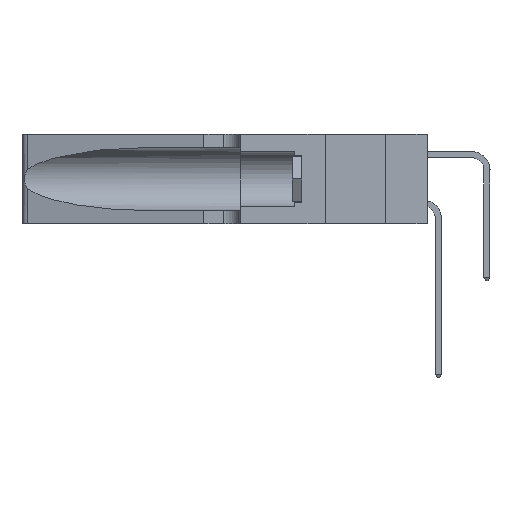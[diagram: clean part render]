
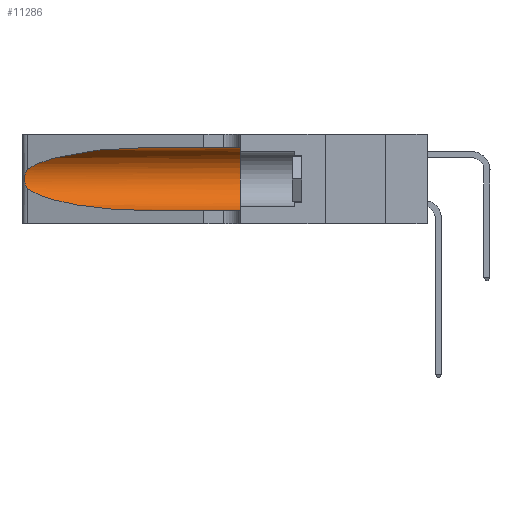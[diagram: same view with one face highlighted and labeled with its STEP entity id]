
A CAD part, left-side view. The second image highlights one B-rep face of the part: STEP entity #11286.
In plain terms, the highlighted cylindrical face has radius 3.308 mm (diameter 6.617 mm), a partial arc.
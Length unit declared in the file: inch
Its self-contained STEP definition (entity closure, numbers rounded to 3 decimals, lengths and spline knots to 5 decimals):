
#25 = ORIENTED_EDGE ( 'NONE', *, *, #1058, .F. ) ;
#624 = CARTESIAN_POINT ( 'NONE',  ( 0.18966, 0.96281, 0.31525 ) ) ;
#1058 = EDGE_CURVE ( 'NONE', #1945, #15296, #40654, .T. ) ;
#1204 = AXIS2_PLACEMENT_3D ( 'NONE', #14312, #21417, #45958 ) ;
#1569 = CARTESIAN_POINT ( 'NONE',  ( 0.25856, 1.23593, 0.16098 ) ) ;
#1945 = VERTEX_POINT ( 'NONE', #13621 ) ;
#3441 = LINE ( 'NONE', #28645, #9776 ) ;
#4288 = CARTESIAN_POINT ( 'NONE',  ( 0.1305, 0.72297, 0.31525 ) ) ;
#5263 = CARTESIAN_POINT ( 'NONE',  ( 0.25639, 1.23186, 0.15144 ) ) ;
#6060 = CARTESIAN_POINT ( 'NONE',  ( 0.1305, 0.72297, 0.05475 ) ) ;
#6554 =( BOUNDED_CURVE ( )  B_SPLINE_CURVE ( 3, ( #9323, #34014, #37522, #16544 ),
 .UNSPECIFIED., .F., .T. ) 
 B_SPLINE_CURVE_WITH_KNOTS ( ( 4, 4 ),
 ( 3.44316, 4.71239 ),
 .UNSPECIFIED. ) 
 CURVE ( )  GEOMETRIC_REPRESENTATION_ITEM ( )  RATIONAL_B_SPLINE_CURVE ( ( 1., 0.87, 0.87, 1. ) ) 
 REPRESENTATION_ITEM ( '' )  );
#7819 = EDGE_CURVE ( 'NONE', #11750, #35818, #38017, .T. ) ;
#8019 = CARTESIAN_POINT ( 'NONE',  ( 0.2373, 1.15595, 0.28018 ) ) ;
#8313 = ORIENTED_EDGE ( 'NONE', *, *, #36297, .T. ) ;
#8961 = CARTESIAN_POINT ( 'NONE',  ( 0.25487, 1.22718, 0.14631 ) ) ;
#9137 = DIRECTION ( 'NONE',  ( 0., 1., 0. ) ) ;
#9323 = CARTESIAN_POINT ( 'NONE',  ( 0.25487, 1.22718, 0.14631 ) ) ;
#9776 = VECTOR ( 'NONE', #11050, 39.37008 ) ;
#9978 = CYLINDRICAL_SURFACE ( 'NONE', #1204, 0.13025 ) ;
#10077 =( BOUNDED_CURVE ( )  B_SPLINE_CURVE ( 3, ( #4288, #624, #8019, #32741 ),
 .UNSPECIFIED., .F., .T. ) 
 B_SPLINE_CURVE_WITH_KNOTS ( ( 4, 4 ),
 ( 1.5708, 2.84003 ),
 .UNSPECIFIED. ) 
 CURVE ( )  GEOMETRIC_REPRESENTATION_ITEM ( )  RATIONAL_B_SPLINE_CURVE ( ( 1., 0.87, 0.87, 1. ) ) 
 REPRESENTATION_ITEM ( '' )  );
#10380 = CARTESIAN_POINT ( 'NONE',  ( 0.1305, 1.61858, 0.31525 ) ) ;
#11050 = DIRECTION ( 'NONE',  ( 0., -1., 0. ) ) ;
#11119 = FACE_OUTER_BOUND ( 'NONE', #19091, .T. ) ;
#11229 = EDGE_CURVE ( 'NONE', #44980, #1945, #32065, .T. ) ;
#11286 = ADVANCED_FACE ( 'NONE', ( #11119 ), #9978, .F. ) ;
#11750 = VERTEX_POINT ( 'NONE', #20463 ) ;
#12424 = CARTESIAN_POINT ( 'NONE',  ( 0.25487, 1.22718, 0.22369 ) ) ;
#13356 = VECTOR ( 'NONE', #28150, 39.37008 ) ;
#13621 = CARTESIAN_POINT ( 'NONE',  ( 0.1305, 0.35, 0.31525 ) ) ;
#14312 = CARTESIAN_POINT ( 'NONE',  ( 0.1305, 1.61858, 0.185 ) ) ;
#15296 = VERTEX_POINT ( 'NONE', #43865 ) ;
#15641 = AXIS2_PLACEMENT_3D ( 'NONE', #30321, #9137, #33827 ) ;
#16033 = CARTESIAN_POINT ( 'NONE',  ( 0.25854, 1.2359, 0.20912 ) ) ;
#16331 = CARTESIAN_POINT ( 'NONE',  ( 0.1305, 0.72297, 0.31525 ) ) ;
#16544 = CARTESIAN_POINT ( 'NONE',  ( 0.1305, 0.72297, 0.05475 ) ) ;
#17543 = CARTESIAN_POINT ( 'NONE',  ( 0.25487, 1.22718, 0.14631 ) ) ;
#19091 = EDGE_LOOP ( 'NONE', ( #41387, #35106, #8313, #22887, #25, #43897 ) ) ;
#19593 = CARTESIAN_POINT ( 'NONE',  ( 0.26075, 1.23896, 0.19203 ) ) ;
#20463 = CARTESIAN_POINT ( 'NONE',  ( 0.25487, 1.22718, 0.22369 ) ) ;
#21417 = DIRECTION ( 'NONE',  ( 0., -1., 0. ) ) ;
#22887 = ORIENTED_EDGE ( 'NONE', *, *, #39846, .T. ) ;
#23118 = CARTESIAN_POINT ( 'NONE',  ( 0.26017, 1.23833, 0.17102 ) ) ;
#26631 = CARTESIAN_POINT ( 'NONE',  ( 0.25789, 1.23486, 0.15765 ) ) ;
#28150 = DIRECTION ( 'NONE',  ( 0., -1., 0. ) ) ;
#28645 = CARTESIAN_POINT ( 'NONE',  ( 0.1305, 1.61858, 0.05475 ) ) ;
#30157 = CARTESIAN_POINT ( 'NONE',  ( 0.25555, 1.22993, 0.14849 ) ) ;
#30321 = CARTESIAN_POINT ( 'NONE',  ( 0.1305, 0.35, 0.185 ) ) ;
#31956 = EDGE_CURVE ( 'NONE', #44980, #11750, #10077, .T. ) ;
#32065 = LINE ( 'NONE', #10380, #13356 ) ;
#32253 = VERTEX_POINT ( 'NONE', #6060 ) ;
#32741 = CARTESIAN_POINT ( 'NONE',  ( 0.25487, 1.22718, 0.22369 ) ) ;
#33355 = CARTESIAN_POINT ( 'NONE',  ( 0.25639, 1.23184, 0.21858 ) ) ;
#33503 = CARTESIAN_POINT ( 'NONE',  ( 0.25555, 1.22994, 0.2215 ) ) ;
#33827 = DIRECTION ( 'NONE',  ( 0., 0., 1. ) ) ;
#34014 = CARTESIAN_POINT ( 'NONE',  ( 0.2373, 1.15595, 0.08982 ) ) ;
#35106 = ORIENTED_EDGE ( 'NONE', *, *, #7819, .T. ) ;
#35818 = VERTEX_POINT ( 'NONE', #17543 ) ;
#36297 = EDGE_CURVE ( 'NONE', #35818, #32253, #6554, .T. ) ;
#37018 = CARTESIAN_POINT ( 'NONE',  ( 0.25787, 1.23484, 0.2124 ) ) ;
#37522 = CARTESIAN_POINT ( 'NONE',  ( 0.18966, 0.96281, 0.05475 ) ) ;
#38017 = B_SPLINE_CURVE_WITH_KNOTS ( 'NONE', 3,
 ( #12424, #33503, #33355, #37018, #16033, #40595, #19593, #44132, #23118, #1569, #26631, #5263, #30157, #8961 ),
 .UNSPECIFIED., .F., .F.,
 ( 4, 2, 2, 2, 2, 2, 4 ),
 ( 0., 0.00027, 0.00053, 0.00107, 0.0016, 0.00187, 0.00214 ),
 .UNSPECIFIED. ) ;
#39846 = EDGE_CURVE ( 'NONE', #32253, #15296, #3441, .T. ) ;
#40595 = CARTESIAN_POINT ( 'NONE',  ( 0.26018, 1.23835, 0.19895 ) ) ;
#40654 = CIRCLE ( 'NONE', #15641, 0.13025 ) ;
#41387 = ORIENTED_EDGE ( 'NONE', *, *, #31956, .T. ) ;
#43865 = CARTESIAN_POINT ( 'NONE',  ( 0.1305, 0.35, 0.05475 ) ) ;
#43897 = ORIENTED_EDGE ( 'NONE', *, *, #11229, .F. ) ;
#44132 = CARTESIAN_POINT ( 'NONE',  ( 0.26075, 1.23896, 0.178 ) ) ;
#44980 = VERTEX_POINT ( 'NONE', #16331 ) ;
#45958 = DIRECTION ( 'NONE',  ( 0., 0., -1. ) ) ;
